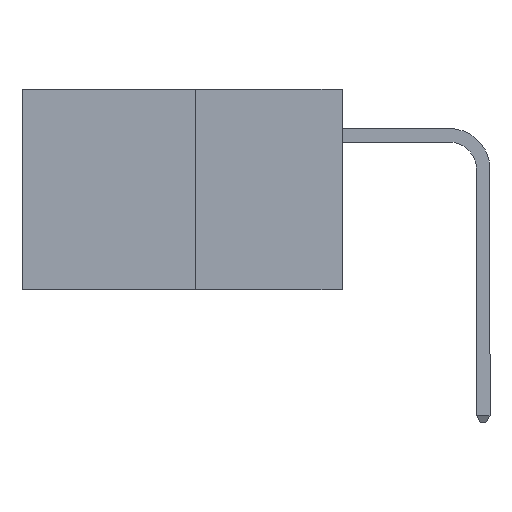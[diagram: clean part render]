
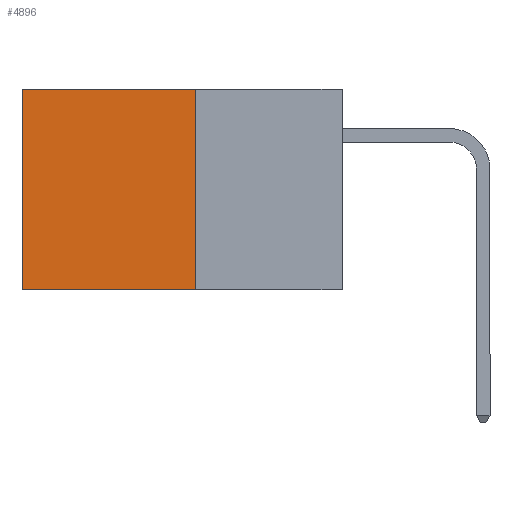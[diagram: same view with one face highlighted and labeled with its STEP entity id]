
A CAD part, left-side view. The second image highlights one B-rep face of the part: STEP entity #4896.
In plain terms, the highlighted planar face has unit normal (-1, 0, 0).
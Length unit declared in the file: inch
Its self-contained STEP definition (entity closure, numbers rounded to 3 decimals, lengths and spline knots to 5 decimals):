
#170 = VECTOR ( 'NONE', #9109, 39.37008 ) ;
#281 = PLANE ( 'NONE',  #8184 ) ;
#1137 = DIRECTION ( 'NONE',  ( 0., 0., -1. ) ) ;
#1138 = EDGE_CURVE ( 'NONE', #1819, #2639, #2097, .T. ) ;
#1157 = ORIENTED_EDGE ( 'NONE', *, *, #5687, .F. ) ;
#1352 = VECTOR ( 'NONE', #7659, 39.37008 ) ;
#1502 = CARTESIAN_POINT ( 'NONE',  ( 0.277, 0.27, 0. ) ) ;
#1695 = DIRECTION ( 'NONE',  ( 0., 0., -1. ) ) ;
#1819 = VERTEX_POINT ( 'NONE', #8188 ) ;
#2028 = FACE_OUTER_BOUND ( 'NONE', #5706, .T. ) ;
#2088 = ORIENTED_EDGE ( 'NONE', *, *, #1138, .T. ) ;
#2097 = LINE ( 'NONE', #10207, #6105 ) ;
#2639 = VERTEX_POINT ( 'NONE', #7372 ) ;
#3745 = CARTESIAN_POINT ( 'NONE',  ( 0.277, 0.27, -0.37 ) ) ;
#4258 = LINE ( 'NONE', #3745, #1352 ) ;
#4744 = ORIENTED_EDGE ( 'NONE', *, *, #9824, .T. ) ;
#4896 = ADVANCED_FACE ( 'NONE', ( #2028 ), #281, .F. ) ;
#4997 = ORIENTED_EDGE ( 'NONE', *, *, #9931, .F. ) ;
#5505 = CARTESIAN_POINT ( 'NONE',  ( 0.277, 0.27, -0.37 ) ) ;
#5687 = EDGE_CURVE ( 'NONE', #8053, #5881, #5755, .T. ) ;
#5706 = EDGE_LOOP ( 'NONE', ( #2088, #4997, #1157, #4744 ) ) ;
#5755 = LINE ( 'NONE', #5505, #9576 ) ;
#5881 = VERTEX_POINT ( 'NONE', #8831 ) ;
#5966 = DIRECTION ( 'NONE',  ( 1., 0., 0. ) ) ;
#6105 = VECTOR ( 'NONE', #1695, 39.37008 ) ;
#6621 = LINE ( 'NONE', #6805, #170 ) ;
#6805 = CARTESIAN_POINT ( 'NONE',  ( 0.277, 0.27, 0. ) ) ;
#7372 = CARTESIAN_POINT ( 'NONE',  ( 0.277, 0.59, -0.37 ) ) ;
#7659 = DIRECTION ( 'NONE',  ( 0., 1., 0. ) ) ;
#8053 = VERTEX_POINT ( 'NONE', #1502 ) ;
#8184 = AXIS2_PLACEMENT_3D ( 'NONE', #9740, #5966, #1137 ) ;
#8188 = CARTESIAN_POINT ( 'NONE',  ( 0.277, 0.59, 0. ) ) ;
#8831 = CARTESIAN_POINT ( 'NONE',  ( 0.277, 0.27, -0.37 ) ) ;
#9109 = DIRECTION ( 'NONE',  ( 0., 1., 0. ) ) ;
#9576 = VECTOR ( 'NONE', #10105, 39.37008 ) ;
#9740 = CARTESIAN_POINT ( 'NONE',  ( 0.277, 0.27, -0.37 ) ) ;
#9824 = EDGE_CURVE ( 'NONE', #8053, #1819, #6621, .T. ) ;
#9931 = EDGE_CURVE ( 'NONE', #5881, #2639, #4258, .T. ) ;
#10105 = DIRECTION ( 'NONE',  ( 0., 0., -1. ) ) ;
#10207 = CARTESIAN_POINT ( 'NONE',  ( 0.277, 0.59, -0.37 ) ) ;
